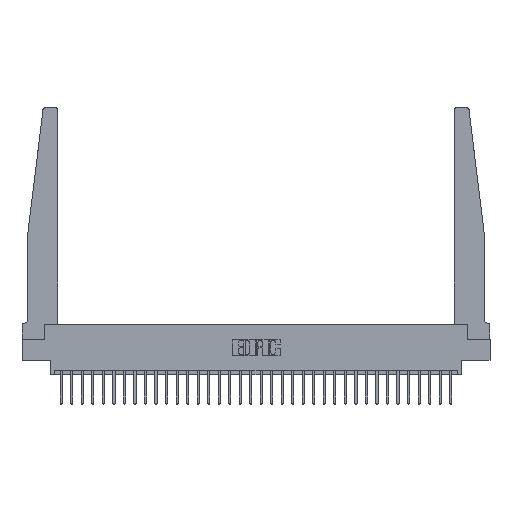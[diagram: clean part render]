
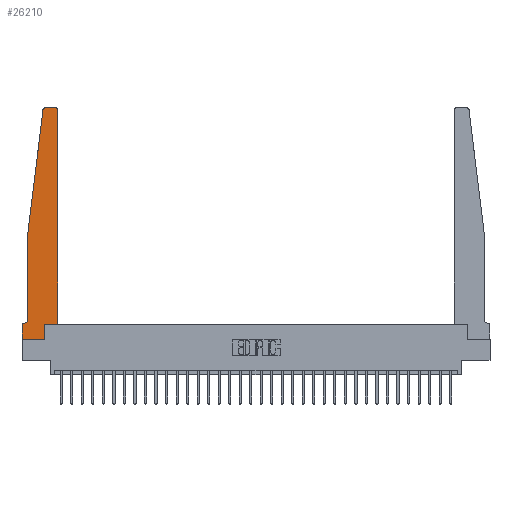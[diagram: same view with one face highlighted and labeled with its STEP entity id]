
A CAD part, top view. The second image highlights one B-rep face of the part: STEP entity #26210.
In plain terms, the highlighted planar face has unit normal (0, 0, 1).
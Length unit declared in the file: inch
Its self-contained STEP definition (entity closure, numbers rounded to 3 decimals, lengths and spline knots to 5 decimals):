
#470 = VECTOR ( 'NONE', #6033, 39.37008 ) ;
#783 = EDGE_CURVE ( 'NONE', #25948, #10745, #7858, .T. ) ;
#2479 = DIRECTION ( 'NONE',  ( 1., 0., 0. ) ) ;
#3466 = VECTOR ( 'NONE', #6777, 39.37008 ) ;
#3649 = CARTESIAN_POINT ( 'NONE',  ( 0., 0.1875, 0.37 ) ) ;
#3822 = CARTESIAN_POINT ( 'NONE',  ( 0.425, 0.18, 0.37 ) ) ;
#4083 = EDGE_CURVE ( 'NONE', #29505, #18156, #27528, .T. ) ;
#4819 = LINE ( 'NONE', #14038, #21974 ) ;
#4823 = ORIENTED_EDGE ( 'NONE', *, *, #5283, .T. ) ;
#5164 = EDGE_CURVE ( 'NONE', #6643, #29505, #8167, .T. ) ;
#5283 = EDGE_CURVE ( 'NONE', #21778, #16327, #27813, .T. ) ;
#5608 = ORIENTED_EDGE ( 'NONE', *, *, #4083, .T. ) ;
#5680 = EDGE_CURVE ( 'NONE', #11911, #22689, #23820, .T. ) ;
#5976 = DIRECTION ( 'NONE',  ( 1., 0., 0. ) ) ;
#6033 = DIRECTION ( 'NONE',  ( 0., -1., 0. ) ) ;
#6489 = VECTOR ( 'NONE', #24035, 39.37008 ) ;
#6643 = VERTEX_POINT ( 'NONE', #21216 ) ;
#6705 = CARTESIAN_POINT ( 'NONE',  ( 0.24675, 2.72367, 0.37 ) ) ;
#6777 = DIRECTION ( 'NONE',  ( -1., 0., 0. ) ) ;
#7605 = FACE_OUTER_BOUND ( 'NONE', #12589, .T. ) ;
#7858 = CIRCLE ( 'NONE', #9896, 0.05 ) ;
#8167 = CIRCLE ( 'NONE', #22216, 0.03 ) ;
#8345 = EDGE_CURVE ( 'NONE', #10745, #13490, #21653, .T. ) ;
#8535 = CARTESIAN_POINT ( 'NONE',  ( 0., 0.1875, 0.37 ) ) ;
#8542 = DIRECTION ( 'NONE',  ( 0., 1., 0. ) ) ;
#8960 = CARTESIAN_POINT ( 'NONE',  ( 0.065, 1.25, 0.37 ) ) ;
#8989 = CARTESIAN_POINT ( 'NONE',  ( 0.395, 2.75, 0.37 ) ) ;
#9101 = EDGE_CURVE ( 'NONE', #24768, #10426, #4819, .T. ) ;
#9242 = VECTOR ( 'NONE', #20371, 39.37008 ) ;
#9896 = AXIS2_PLACEMENT_3D ( 'NONE', #20817, #29756, #21339 ) ;
#10426 = VERTEX_POINT ( 'NONE', #3822 ) ;
#10720 = VECTOR ( 'NONE', #17390, 39.37008 ) ;
#10745 = VERTEX_POINT ( 'NONE', #14213 ) ;
#10746 = VECTOR ( 'NONE', #27579, 39.37008 ) ;
#10832 = CARTESIAN_POINT ( 'NONE',  ( 0.395, 2.72, 0.37 ) ) ;
#11162 = VECTOR ( 'NONE', #28245, 39.37008 ) ;
#11203 = CARTESIAN_POINT ( 'NONE',  ( 0.27653, 2.72, 0.37 ) ) ;
#11757 = EDGE_CURVE ( 'NONE', #18156, #21778, #28335, .T. ) ;
#11911 = VERTEX_POINT ( 'NONE', #25625 ) ;
#12210 = CARTESIAN_POINT ( 'NONE',  ( 0.065, 1.25, 0.37 ) ) ;
#12589 = EDGE_LOOP ( 'NONE', ( #5608, #20941, #4823, #25086, #19796, #18535, #14478, #13450, #21601, #25935, #15206, #20028 ) ) ;
#13175 = DIRECTION ( 'NONE',  ( 1., 0., 0. ) ) ;
#13450 = ORIENTED_EDGE ( 'NONE', *, *, #5680, .T. ) ;
#13459 = LINE ( 'NONE', #19336, #6489 ) ;
#13490 = VERTEX_POINT ( 'NONE', #8535 ) ;
#13548 = DIRECTION ( 'NONE',  ( 1., 0., 0. ) ) ;
#13702 = LINE ( 'NONE', #22264, #470 ) ;
#14038 = CARTESIAN_POINT ( 'NONE',  ( 0.425, 0.18, 0.37 ) ) ;
#14213 = CARTESIAN_POINT ( 'NONE',  ( 0.015, 0.1875, 0.37 ) ) ;
#14478 = ORIENTED_EDGE ( 'NONE', *, *, #29308, .T. ) ;
#15206 = ORIENTED_EDGE ( 'NONE', *, *, #23684, .T. ) ;
#15281 = EDGE_CURVE ( 'NONE', #22689, #24768, #13459, .T. ) ;
#15587 = CARTESIAN_POINT ( 'NONE',  ( 0.425, 0.18, 0.37 ) ) ;
#16327 = VERTEX_POINT ( 'NONE', #17156 ) ;
#17156 = CARTESIAN_POINT ( 'NONE',  ( 0.065, 1.25, 0.37 ) ) ;
#17390 = DIRECTION ( 'NONE',  ( 1., 0., 0. ) ) ;
#17613 = PLANE ( 'NONE',  #17695 ) ;
#17695 = AXIS2_PLACEMENT_3D ( 'NONE', #3649, #19953, #5976 ) ;
#18156 = VERTEX_POINT ( 'NONE', #26618 ) ;
#18535 = ORIENTED_EDGE ( 'NONE', *, *, #8345, .T. ) ;
#19336 = CARTESIAN_POINT ( 'NONE',  ( 0.2605, 0.18, 0.37 ) ) ;
#19796 = ORIENTED_EDGE ( 'NONE', *, *, #783, .T. ) ;
#19953 = DIRECTION ( 'NONE',  ( 0., 0., 1. ) ) ;
#20028 = ORIENTED_EDGE ( 'NONE', *, *, #5164, .T. ) ;
#20371 = DIRECTION ( 'NONE',  ( -1., 0., 0. ) ) ;
#20817 = CARTESIAN_POINT ( 'NONE',  ( 0.015, 0.2375, 0.37 ) ) ;
#20941 = ORIENTED_EDGE ( 'NONE', *, *, #11757, .T. ) ;
#21216 = CARTESIAN_POINT ( 'NONE',  ( 0.425, 2.72, 0.37 ) ) ;
#21339 = DIRECTION ( 'NONE',  ( -1., 0., 0. ) ) ;
#21601 = ORIENTED_EDGE ( 'NONE', *, *, #15281, .T. ) ;
#21653 = LINE ( 'NONE', #29635, #9242 ) ;
#21778 = VERTEX_POINT ( 'NONE', #6705 ) ;
#21974 = VECTOR ( 'NONE', #2479, 39.37008 ) ;
#22216 = AXIS2_PLACEMENT_3D ( 'NONE', #10832, #27094, #13175 ) ;
#22264 = CARTESIAN_POINT ( 'NONE',  ( 0., 0., 0.37 ) ) ;
#22689 = VERTEX_POINT ( 'NONE', #24084 ) ;
#23086 = CARTESIAN_POINT ( 'NONE',  ( 0.25, 2.75, 0.37 ) ) ;
#23684 = EDGE_CURVE ( 'NONE', #10426, #6643, #24530, .T. ) ;
#23799 = VECTOR ( 'NONE', #8542, 39.37008 ) ;
#23820 = LINE ( 'NONE', #29001, #10720 ) ;
#24035 = DIRECTION ( 'NONE',  ( 0., 1., 0. ) ) ;
#24084 = CARTESIAN_POINT ( 'NONE',  ( 0.2605, 0., 0.37 ) ) ;
#24274 = LINE ( 'NONE', #12210, #11162 ) ;
#24530 = LINE ( 'NONE', #15587, #23799 ) ;
#24768 = VERTEX_POINT ( 'NONE', #29255 ) ;
#25086 = ORIENTED_EDGE ( 'NONE', *, *, #29132, .T. ) ;
#25238 = AXIS2_PLACEMENT_3D ( 'NONE', #11203, #27459, #13548 ) ;
#25625 = CARTESIAN_POINT ( 'NONE',  ( 0., 0., 0.37 ) ) ;
#25935 = ORIENTED_EDGE ( 'NONE', *, *, #9101, .T. ) ;
#25948 = VERTEX_POINT ( 'NONE', #28000 ) ;
#26210 = ADVANCED_FACE ( 'NONE', ( #7605 ), #17613, .T. ) ;
#26618 = CARTESIAN_POINT ( 'NONE',  ( 0.27653, 2.75, 0.37 ) ) ;
#27094 = DIRECTION ( 'NONE',  ( 0., 0., 1. ) ) ;
#27459 = DIRECTION ( 'NONE',  ( 0., 0., 1. ) ) ;
#27528 = LINE ( 'NONE', #23086, #3466 ) ;
#27579 = DIRECTION ( 'NONE',  ( -0.122, -0.992, 0. ) ) ;
#27813 = LINE ( 'NONE', #8960, #10746 ) ;
#28000 = CARTESIAN_POINT ( 'NONE',  ( 0.065, 0.2375, 0.37 ) ) ;
#28245 = DIRECTION ( 'NONE',  ( 0., -1., 0. ) ) ;
#28335 = CIRCLE ( 'NONE', #25238, 0.03 ) ;
#29001 = CARTESIAN_POINT ( 'NONE',  ( 0., 0., 0.37 ) ) ;
#29132 = EDGE_CURVE ( 'NONE', #16327, #25948, #24274, .T. ) ;
#29255 = CARTESIAN_POINT ( 'NONE',  ( 0.2605, 0.18, 0.37 ) ) ;
#29308 = EDGE_CURVE ( 'NONE', #13490, #11911, #13702, .T. ) ;
#29505 = VERTEX_POINT ( 'NONE', #8989 ) ;
#29635 = CARTESIAN_POINT ( 'NONE',  ( 0.065, 0.1875, 0.37 ) ) ;
#29756 = DIRECTION ( 'NONE',  ( 0., 0., -1. ) ) ;
